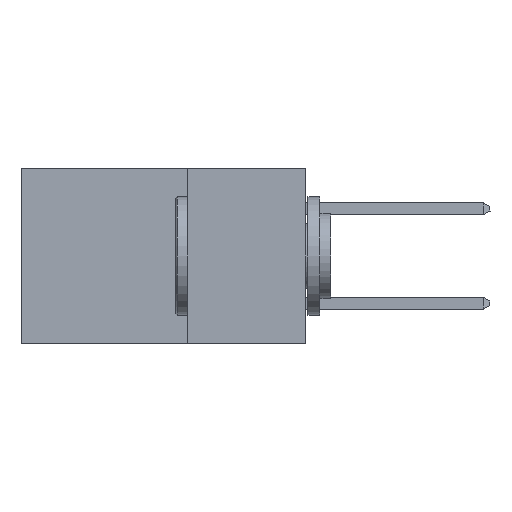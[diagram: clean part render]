
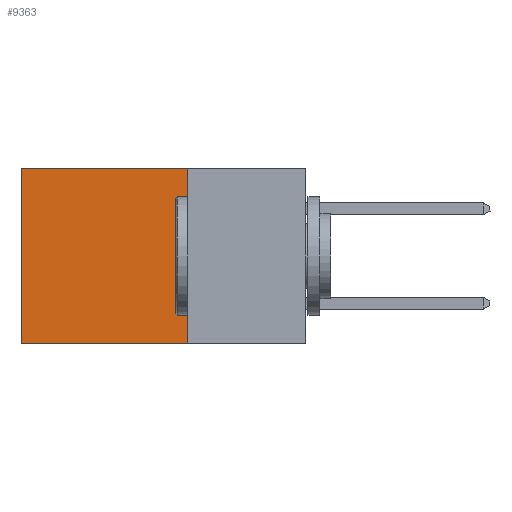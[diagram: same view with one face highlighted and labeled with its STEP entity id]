
A CAD part, left-side view. The second image highlights one B-rep face of the part: STEP entity #9363.
In plain terms, the highlighted planar face has unit normal (-1, 0, 0).
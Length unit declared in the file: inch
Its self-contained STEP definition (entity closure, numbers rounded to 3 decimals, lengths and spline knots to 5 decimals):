
#71 = EDGE_CURVE ( 'NONE', #5952, #4369, #2992, .T. ) ;
#140 = LINE ( 'NONE', #12575, #6330 ) ;
#762 = VECTOR ( 'NONE', #2886, 39.37008 ) ;
#1108 = DIRECTION ( 'NONE',  ( 0., 0., -1. ) ) ;
#1175 = LINE ( 'NONE', #5159, #1821 ) ;
#1821 = VECTOR ( 'NONE', #7457, 39.37008 ) ;
#1967 = AXIS2_PLACEMENT_3D ( 'NONE', #9228, #12315, #1108 ) ;
#2068 = ORIENTED_EDGE ( 'NONE', *, *, #71, .F. ) ;
#2084 = CARTESIAN_POINT ( 'NONE',  ( 0.298, 0.25, 0. ) ) ;
#2332 = CARTESIAN_POINT ( 'NONE',  ( 0.298, 0.6, 0. ) ) ;
#2808 = CARTESIAN_POINT ( 'NONE',  ( 0.298, 0.25, 0. ) ) ;
#2886 = DIRECTION ( 'NONE',  ( 0., 1., 0. ) ) ;
#2992 = LINE ( 'NONE', #9907, #762 ) ;
#3294 = LINE ( 'NONE', #2808, #13189 ) ;
#4369 = VERTEX_POINT ( 'NONE', #8346 ) ;
#4648 = ORIENTED_EDGE ( 'NONE', *, *, #8234, .T. ) ;
#4754 = ORIENTED_EDGE ( 'NONE', *, *, #10631, .T. ) ;
#4827 = EDGE_CURVE ( 'NONE', #4953, #5952, #3294, .T. ) ;
#4953 = VERTEX_POINT ( 'NONE', #2084 ) ;
#5159 = CARTESIAN_POINT ( 'NONE',  ( 0.298, 0.6, 0. ) ) ;
#5197 = PLANE ( 'NONE',  #1967 ) ;
#5952 = VERTEX_POINT ( 'NONE', #8299 ) ;
#6120 = ORIENTED_EDGE ( 'NONE', *, *, #4827, .F. ) ;
#6330 = VECTOR ( 'NONE', #6446, 39.37008 ) ;
#6446 = DIRECTION ( 'NONE',  ( 0., 1., 0. ) ) ;
#7457 = DIRECTION ( 'NONE',  ( 0., 0., -1. ) ) ;
#7526 = EDGE_LOOP ( 'NONE', ( #4754, #2068, #6120, #4648 ) ) ;
#8234 = EDGE_CURVE ( 'NONE', #4953, #8786, #140, .T. ) ;
#8299 = CARTESIAN_POINT ( 'NONE',  ( 0.298, 0.25, -0.37 ) ) ;
#8346 = CARTESIAN_POINT ( 'NONE',  ( 0.298, 0.6, -0.37 ) ) ;
#8400 = FACE_OUTER_BOUND ( 'NONE', #7526, .T. ) ;
#8786 = VERTEX_POINT ( 'NONE', #2332 ) ;
#9228 = CARTESIAN_POINT ( 'NONE',  ( 0.298, 0.25, 0. ) ) ;
#9363 = ADVANCED_FACE ( 'NONE', ( #8400 ), #5197, .F. ) ;
#9907 = CARTESIAN_POINT ( 'NONE',  ( 0.298, 0.25, -0.37 ) ) ;
#10631 = EDGE_CURVE ( 'NONE', #8786, #4369, #1175, .T. ) ;
#12140 = DIRECTION ( 'NONE',  ( 0., 0., -1. ) ) ;
#12315 = DIRECTION ( 'NONE',  ( 1., 0., 0. ) ) ;
#12575 = CARTESIAN_POINT ( 'NONE',  ( 0.298, 0.25, 0. ) ) ;
#13189 = VECTOR ( 'NONE', #12140, 39.37008 ) ;
